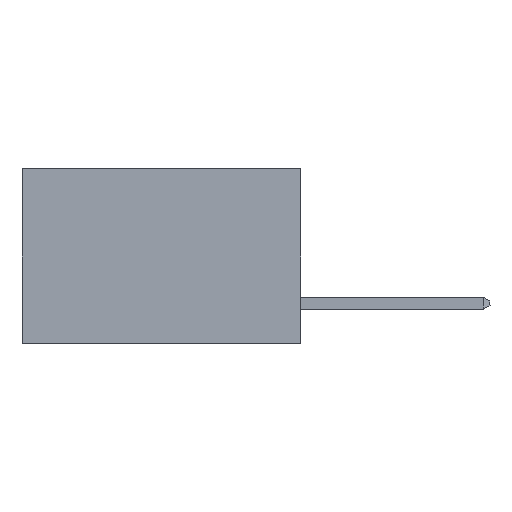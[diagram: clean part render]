
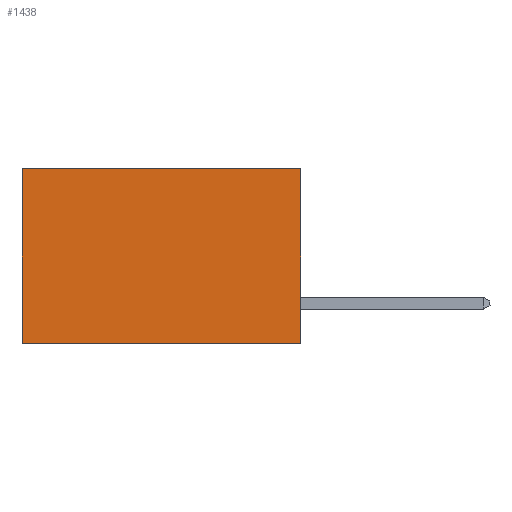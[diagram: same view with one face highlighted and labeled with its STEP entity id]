
A CAD part, left-side view. The second image highlights one B-rep face of the part: STEP entity #1438.
In plain terms, the highlighted planar face has unit normal (-1, 0, 0).
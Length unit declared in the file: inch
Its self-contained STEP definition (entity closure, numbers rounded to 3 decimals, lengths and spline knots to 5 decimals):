
#130 = CARTESIAN_POINT ( 'NONE',  ( 0.277, 0., 0. ) ) ;
#695 = VERTEX_POINT ( 'NONE', #130 ) ;
#1324 = DIRECTION ( 'NONE',  ( 0., 0., -1. ) ) ;
#1438 = ADVANCED_FACE ( 'NONE', ( #9884 ), #10193, .F. ) ;
#1448 = DIRECTION ( 'NONE',  ( 1., 0., 0. ) ) ;
#1458 = DIRECTION ( 'NONE',  ( 0., 0., -1. ) ) ;
#1657 = CARTESIAN_POINT ( 'NONE',  ( 0.277, 0.59, 0. ) ) ;
#1833 = EDGE_CURVE ( 'NONE', #695, #7961, #8272, .T. ) ;
#2239 = EDGE_CURVE ( 'NONE', #7961, #4879, #8566, .T. ) ;
#2830 = VECTOR ( 'NONE', #1324, 39.37008 ) ;
#3733 = VECTOR ( 'NONE', #10248, 39.37008 ) ;
#3772 = ORIENTED_EDGE ( 'NONE', *, *, #6661, .T. ) ;
#3827 = AXIS2_PLACEMENT_3D ( 'NONE', #10273, #1448, #1458 ) ;
#4879 = VERTEX_POINT ( 'NONE', #9491 ) ;
#5027 = ORIENTED_EDGE ( 'NONE', *, *, #1833, .F. ) ;
#5461 = LINE ( 'NONE', #8077, #2830 ) ;
#5785 = VECTOR ( 'NONE', #6232, 39.37008 ) ;
#6072 = VECTOR ( 'NONE', #6396, 39.37008 ) ;
#6161 = CARTESIAN_POINT ( 'NONE',  ( 0.277, 0., -0.37 ) ) ;
#6232 = DIRECTION ( 'NONE',  ( 0., 0., -1. ) ) ;
#6281 = VERTEX_POINT ( 'NONE', #1657 ) ;
#6396 = DIRECTION ( 'NONE',  ( 0., 1., 0. ) ) ;
#6661 = EDGE_CURVE ( 'NONE', #695, #6281, #11209, .T. ) ;
#6972 = CARTESIAN_POINT ( 'NONE',  ( 0.277, 0., -0.37 ) ) ;
#7961 = VERTEX_POINT ( 'NONE', #6161 ) ;
#8077 = CARTESIAN_POINT ( 'NONE',  ( 0.277, 0.59, -0.37 ) ) ;
#8230 = ORIENTED_EDGE ( 'NONE', *, *, #10487, .T. ) ;
#8272 = LINE ( 'NONE', #11148, #5785 ) ;
#8566 = LINE ( 'NONE', #6972, #6072 ) ;
#8665 = CARTESIAN_POINT ( 'NONE',  ( 0.277, 0., 0. ) ) ;
#9491 = CARTESIAN_POINT ( 'NONE',  ( 0.277, 0.59, -0.37 ) ) ;
#9738 = ORIENTED_EDGE ( 'NONE', *, *, #2239, .F. ) ;
#9884 = FACE_OUTER_BOUND ( 'NONE', #10583, .T. ) ;
#10193 = PLANE ( 'NONE',  #3827 ) ;
#10248 = DIRECTION ( 'NONE',  ( 0., 1., 0. ) ) ;
#10273 = CARTESIAN_POINT ( 'NONE',  ( 0.277, 0., -0.37 ) ) ;
#10487 = EDGE_CURVE ( 'NONE', #6281, #4879, #5461, .T. ) ;
#10583 = EDGE_LOOP ( 'NONE', ( #8230, #9738, #5027, #3772 ) ) ;
#11148 = CARTESIAN_POINT ( 'NONE',  ( 0.277, 0., -0.37 ) ) ;
#11209 = LINE ( 'NONE', #8665, #3733 ) ;
